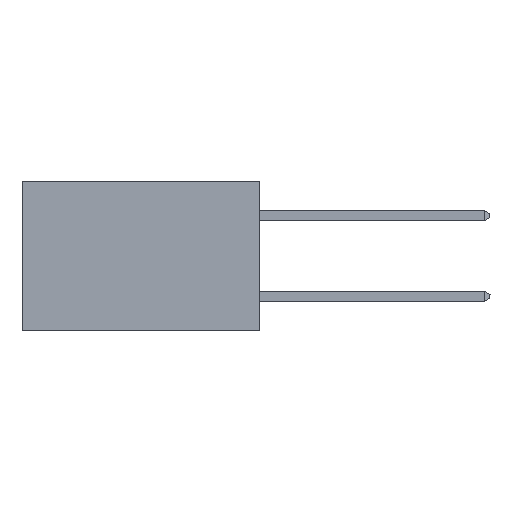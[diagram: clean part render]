
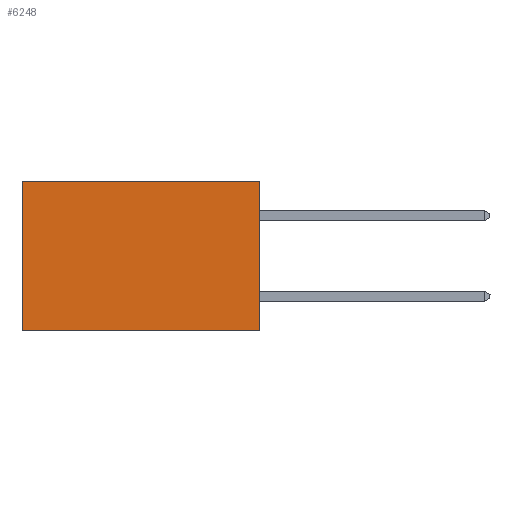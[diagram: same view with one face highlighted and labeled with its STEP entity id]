
A CAD part, left-side view. The second image highlights one B-rep face of the part: STEP entity #6248.
In plain terms, the highlighted planar face has unit normal (-1, 0, 0).
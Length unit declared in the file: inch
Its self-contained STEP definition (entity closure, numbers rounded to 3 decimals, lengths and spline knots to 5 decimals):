
#211 = CARTESIAN_POINT ( 'NONE',  ( 0.277, 0., -0.37 ) ) ;
#707 = LINE ( 'NONE', #1000, #4508 ) ;
#877 = DIRECTION ( 'NONE',  ( 0., 0., -1. ) ) ;
#895 = VECTOR ( 'NONE', #2029, 39.37008 ) ;
#1000 = CARTESIAN_POINT ( 'NONE',  ( 0.277, 0., -0.37 ) ) ;
#1013 = LINE ( 'NONE', #4195, #6585 ) ;
#1319 = CARTESIAN_POINT ( 'NONE',  ( 0.277, 0., 0. ) ) ;
#1696 = CARTESIAN_POINT ( 'NONE',  ( 0.277, 0., 0. ) ) ;
#1832 = ORIENTED_EDGE ( 'NONE', *, *, #3459, .T. ) ;
#2029 = DIRECTION ( 'NONE',  ( 0., 1., 0. ) ) ;
#2059 = VERTEX_POINT ( 'NONE', #1319 ) ;
#2263 = AXIS2_PLACEMENT_3D ( 'NONE', #7561, #7824, #7544 ) ;
#2356 = ORIENTED_EDGE ( 'NONE', *, *, #4619, .F. ) ;
#2564 = ORIENTED_EDGE ( 'NONE', *, *, #4633, .F. ) ;
#2882 = DIRECTION ( 'NONE',  ( 0., 0., -1. ) ) ;
#2999 = LINE ( 'NONE', #8485, #6744 ) ;
#3336 = EDGE_CURVE ( 'NONE', #2059, #5041, #6711, .T. ) ;
#3459 = EDGE_CURVE ( 'NONE', #5041, #7876, #1013, .T. ) ;
#4012 = ORIENTED_EDGE ( 'NONE', *, *, #3336, .T. ) ;
#4195 = CARTESIAN_POINT ( 'NONE',  ( 0.277, 0.59, -0.37 ) ) ;
#4508 = VECTOR ( 'NONE', #877, 39.37008 ) ;
#4591 = VERTEX_POINT ( 'NONE', #211 ) ;
#4619 = EDGE_CURVE ( 'NONE', #4591, #7876, #2999, .T. ) ;
#4633 = EDGE_CURVE ( 'NONE', #2059, #4591, #707, .T. ) ;
#5041 = VERTEX_POINT ( 'NONE', #8420 ) ;
#6248 = ADVANCED_FACE ( 'NONE', ( #7111 ), #8081, .F. ) ;
#6585 = VECTOR ( 'NONE', #2882, 39.37008 ) ;
#6711 = LINE ( 'NONE', #1696, #895 ) ;
#6744 = VECTOR ( 'NONE', #8469, 39.37008 ) ;
#7111 = FACE_OUTER_BOUND ( 'NONE', #8351, .T. ) ;
#7263 = CARTESIAN_POINT ( 'NONE',  ( 0.277, 0.59, -0.37 ) ) ;
#7544 = DIRECTION ( 'NONE',  ( 0., 0., -1. ) ) ;
#7561 = CARTESIAN_POINT ( 'NONE',  ( 0.277, 0., -0.37 ) ) ;
#7824 = DIRECTION ( 'NONE',  ( 1., 0., 0. ) ) ;
#7876 = VERTEX_POINT ( 'NONE', #7263 ) ;
#8081 = PLANE ( 'NONE',  #2263 ) ;
#8351 = EDGE_LOOP ( 'NONE', ( #1832, #2356, #2564, #4012 ) ) ;
#8420 = CARTESIAN_POINT ( 'NONE',  ( 0.277, 0.59, 0. ) ) ;
#8469 = DIRECTION ( 'NONE',  ( 0., 1., 0. ) ) ;
#8485 = CARTESIAN_POINT ( 'NONE',  ( 0.277, 0., -0.37 ) ) ;
